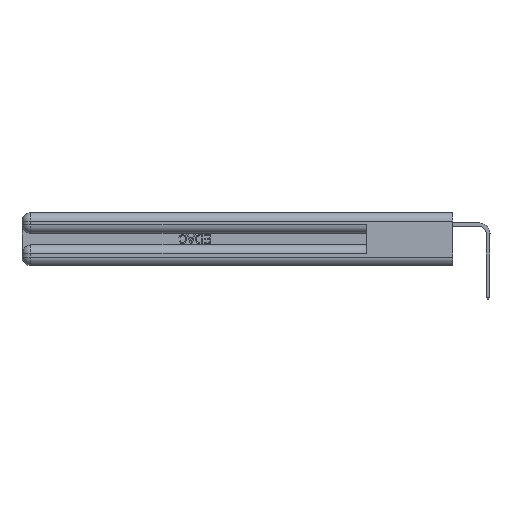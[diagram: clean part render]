
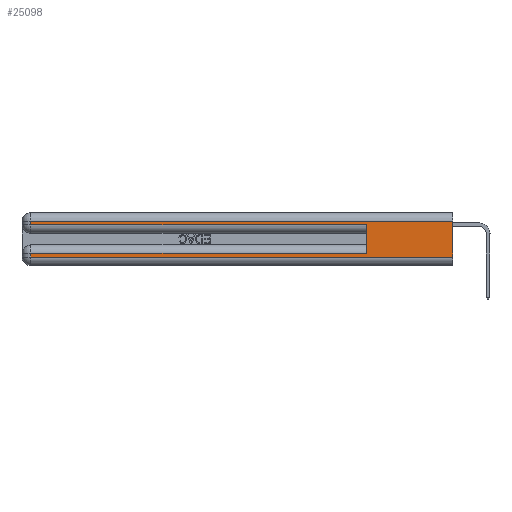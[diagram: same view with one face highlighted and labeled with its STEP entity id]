
A CAD part, left-side view. The second image highlights one B-rep face of the part: STEP entity #25098.
In plain terms, the highlighted planar face has unit normal (-1, 0, 0).
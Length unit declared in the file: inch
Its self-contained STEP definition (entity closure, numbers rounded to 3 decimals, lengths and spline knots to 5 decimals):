
#235 = DIRECTION ( 'NONE',  ( 0., -1., 0. ) ) ;
#718 = AXIS2_PLACEMENT_3D ( 'NONE', #7975, #4633, #28920 ) ;
#2136 = CARTESIAN_POINT ( 'NONE',  ( 0., 0.6, 0.085 ) ) ;
#2164 = VERTEX_POINT ( 'NONE', #16970 ) ;
#2606 = DIRECTION ( 'NONE',  ( 0., 0., 1. ) ) ;
#2713 = ORIENTED_EDGE ( 'NONE', *, *, #6111, .F. ) ;
#2798 = LINE ( 'NONE', #26897, #20212 ) ;
#3489 = VECTOR ( 'NONE', #17839, 39.37008 ) ;
#3686 = VECTOR ( 'NONE', #17643, 39.37008 ) ;
#3860 = EDGE_CURVE ( 'NONE', #2164, #4235, #11589, .T. ) ;
#4189 = CARTESIAN_POINT ( 'NONE',  ( 0., 0., 0.085 ) ) ;
#4235 = VERTEX_POINT ( 'NONE', #5682 ) ;
#4324 = DIRECTION ( 'NONE',  ( 0., -1., 0. ) ) ;
#4633 = DIRECTION ( 'NONE',  ( 1., 0., 0. ) ) ;
#5155 = CARTESIAN_POINT ( 'NONE',  ( 0., 2.94, 0.31 ) ) ;
#5381 = CARTESIAN_POINT ( 'NONE',  ( 0., 2.94, 0.37 ) ) ;
#5682 = CARTESIAN_POINT ( 'NONE',  ( 0., 0., 0.06 ) ) ;
#6111 = EDGE_CURVE ( 'NONE', #11651, #10540, #2798, .T. ) ;
#7701 = EDGE_CURVE ( 'NONE', #31735, #35184, #31372, .T. ) ;
#7975 = CARTESIAN_POINT ( 'NONE',  ( 0., 0., 0.37 ) ) ;
#8373 = DIRECTION ( 'NONE',  ( 0., 1., 0. ) ) ;
#9022 = EDGE_CURVE ( 'NONE', #15365, #10540, #21587, .T. ) ;
#10239 = ORIENTED_EDGE ( 'NONE', *, *, #3860, .F. ) ;
#10540 = VERTEX_POINT ( 'NONE', #31184 ) ;
#11474 = FACE_OUTER_BOUND ( 'NONE', #31451, .T. ) ;
#11589 = LINE ( 'NONE', #14145, #3489 ) ;
#11651 = VERTEX_POINT ( 'NONE', #2136 ) ;
#12071 = ORIENTED_EDGE ( 'NONE', *, *, #7701, .T. ) ;
#13108 = EDGE_CURVE ( 'NONE', #19504, #15365, #26054, .T. ) ;
#14101 = CARTESIAN_POINT ( 'NONE',  ( 0., 2.94, 0.37 ) ) ;
#14145 = CARTESIAN_POINT ( 'NONE',  ( 0., 0., 0.37 ) ) ;
#14411 = VECTOR ( 'NONE', #8373, 39.37008 ) ;
#15365 = VERTEX_POINT ( 'NONE', #39621 ) ;
#16970 = CARTESIAN_POINT ( 'NONE',  ( 0., 0., 0.31 ) ) ;
#17643 = DIRECTION ( 'NONE',  ( 0., 0., -1. ) ) ;
#17839 = DIRECTION ( 'NONE',  ( 0., 0., -1. ) ) ;
#19504 = VERTEX_POINT ( 'NONE', #5155 ) ;
#20212 = VECTOR ( 'NONE', #2606, 39.37008 ) ;
#21587 = LINE ( 'NONE', #25159, #29686 ) ;
#22262 = CARTESIAN_POINT ( 'NONE',  ( 0., 0., 0.31 ) ) ;
#22865 = EDGE_CURVE ( 'NONE', #35184, #4235, #41011, .T. ) ;
#23456 = ORIENTED_EDGE ( 'NONE', *, *, #32200, .T. ) ;
#25030 = DIRECTION ( 'NONE',  ( 0., 1., 0. ) ) ;
#25098 = ADVANCED_FACE ( 'NONE', ( #11474 ), #25474, .F. ) ;
#25159 = CARTESIAN_POINT ( 'NONE',  ( 0., 0., 0.285 ) ) ;
#25474 = PLANE ( 'NONE',  #718 ) ;
#26054 = LINE ( 'NONE', #5381, #35238 ) ;
#26068 = ORIENTED_EDGE ( 'NONE', *, *, #22865, .T. ) ;
#26897 = CARTESIAN_POINT ( 'NONE',  ( 0., 0.6, 0.145 ) ) ;
#28390 = VECTOR ( 'NONE', #25030, 39.37008 ) ;
#28920 = DIRECTION ( 'NONE',  ( 0., 0., -1. ) ) ;
#29686 = VECTOR ( 'NONE', #4324, 39.37008 ) ;
#31184 = CARTESIAN_POINT ( 'NONE',  ( 0., 0.6, 0.285 ) ) ;
#31372 = LINE ( 'NONE', #14101, #3686 ) ;
#31451 = EDGE_LOOP ( 'NONE', ( #10239, #34640, #43160, #41707, #2713, #23456, #12071, #26068 ) ) ;
#31735 = VERTEX_POINT ( 'NONE', #33400 ) ;
#31830 = VECTOR ( 'NONE', #235, 39.37008 ) ;
#32200 = EDGE_CURVE ( 'NONE', #11651, #31735, #37605, .T. ) ;
#32914 = LINE ( 'NONE', #22262, #14411 ) ;
#33150 = DIRECTION ( 'NONE',  ( 0., 0., -1. ) ) ;
#33400 = CARTESIAN_POINT ( 'NONE',  ( 0., 2.94, 0.085 ) ) ;
#34640 = ORIENTED_EDGE ( 'NONE', *, *, #43763, .T. ) ;
#35184 = VERTEX_POINT ( 'NONE', #36146 ) ;
#35238 = VECTOR ( 'NONE', #33150, 39.37008 ) ;
#36146 = CARTESIAN_POINT ( 'NONE',  ( 0., 2.94, 0.06 ) ) ;
#37605 = LINE ( 'NONE', #4189, #28390 ) ;
#39621 = CARTESIAN_POINT ( 'NONE',  ( 0., 2.94, 0.285 ) ) ;
#41011 = LINE ( 'NONE', #44930, #31830 ) ;
#41707 = ORIENTED_EDGE ( 'NONE', *, *, #9022, .T. ) ;
#43160 = ORIENTED_EDGE ( 'NONE', *, *, #13108, .T. ) ;
#43763 = EDGE_CURVE ( 'NONE', #2164, #19504, #32914, .T. ) ;
#44930 = CARTESIAN_POINT ( 'NONE',  ( 0., 0., 0.06 ) ) ;
